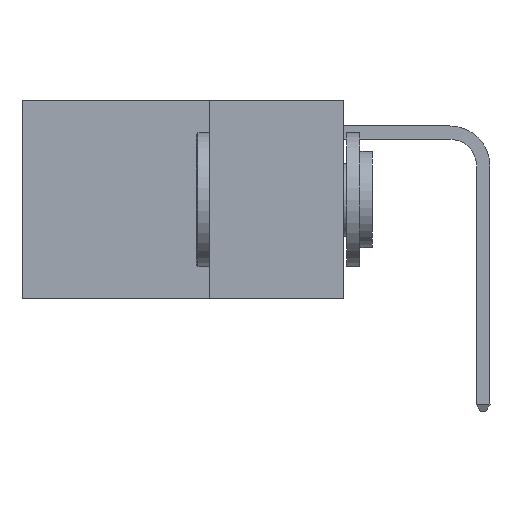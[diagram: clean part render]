
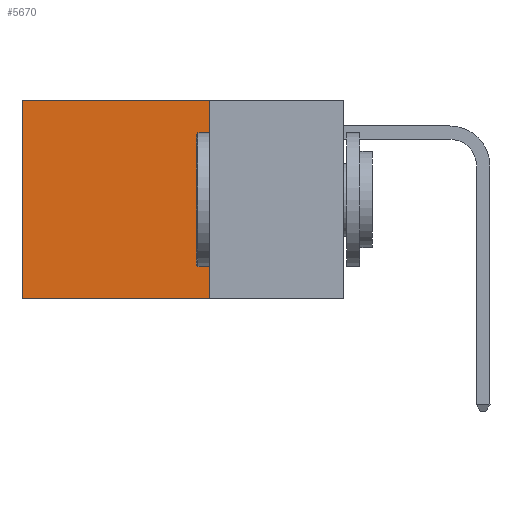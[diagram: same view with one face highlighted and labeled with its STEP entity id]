
A CAD part, left-side view. The second image highlights one B-rep face of the part: STEP entity #5670.
In plain terms, the highlighted planar face has unit normal (-1, 0, 0).
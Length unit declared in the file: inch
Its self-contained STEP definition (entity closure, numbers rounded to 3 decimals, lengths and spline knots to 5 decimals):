
#886 = DIRECTION ( 'NONE',  ( 0., 0., -1. ) ) ;
#1220 = EDGE_CURVE ( 'NONE', #5242, #13661, #16678, .T. ) ;
#1494 = CARTESIAN_POINT ( 'NONE',  ( 0.2625, 0.6, -0.37 ) ) ;
#1855 = FACE_OUTER_BOUND ( 'NONE', #3668, .T. ) ;
#3451 = ORIENTED_EDGE ( 'NONE', *, *, #4221, .T. ) ;
#3668 = EDGE_LOOP ( 'NONE', ( #5160, #16306, #18727, #3451 ) ) ;
#4221 = EDGE_CURVE ( 'NONE', #19881, #21653, #9118, .T. ) ;
#4282 = VECTOR ( 'NONE', #22397, 39.37008 ) ;
#5160 = ORIENTED_EDGE ( 'NONE', *, *, #14125, .T. ) ;
#5242 = VERTEX_POINT ( 'NONE', #20139 ) ;
#5670 = ADVANCED_FACE ( 'NONE', ( #1855 ), #11281, .F. ) ;
#5891 = CARTESIAN_POINT ( 'NONE',  ( 0.2625, 0.25, 0. ) ) ;
#5895 = DIRECTION ( 'NONE',  ( 1., 0., 0. ) ) ;
#7608 = CARTESIAN_POINT ( 'NONE',  ( 0.2625, 0.25, -0.37 ) ) ;
#8099 = LINE ( 'NONE', #20330, #16848 ) ;
#8578 = CARTESIAN_POINT ( 'NONE',  ( 0.2625, 0.25, 0. ) ) ;
#8615 = EDGE_CURVE ( 'NONE', #19881, #5242, #8099, .T. ) ;
#9118 = LINE ( 'NONE', #8578, #4282 ) ;
#10385 = DIRECTION ( 'NONE',  ( 0., 1., 0. ) ) ;
#10437 = LINE ( 'NONE', #22069, #15049 ) ;
#11281 = PLANE ( 'NONE',  #16827 ) ;
#13661 = VERTEX_POINT ( 'NONE', #1494 ) ;
#14125 = EDGE_CURVE ( 'NONE', #21653, #13661, #10437, .T. ) ;
#15049 = VECTOR ( 'NONE', #886, 39.37008 ) ;
#16159 = VECTOR ( 'NONE', #10385, 39.37008 ) ;
#16306 = ORIENTED_EDGE ( 'NONE', *, *, #1220, .F. ) ;
#16457 = CARTESIAN_POINT ( 'NONE',  ( 0.2625, 0.25, 0. ) ) ;
#16563 = CARTESIAN_POINT ( 'NONE',  ( 0.2625, 0.6, 0. ) ) ;
#16678 = LINE ( 'NONE', #7608, #16159 ) ;
#16827 = AXIS2_PLACEMENT_3D ( 'NONE', #16457, #5895, #18172 ) ;
#16848 = VECTOR ( 'NONE', #22030, 39.37008 ) ;
#18172 = DIRECTION ( 'NONE',  ( 0., 0., -1. ) ) ;
#18727 = ORIENTED_EDGE ( 'NONE', *, *, #8615, .F. ) ;
#19881 = VERTEX_POINT ( 'NONE', #5891 ) ;
#20139 = CARTESIAN_POINT ( 'NONE',  ( 0.2625, 0.25, -0.37 ) ) ;
#20330 = CARTESIAN_POINT ( 'NONE',  ( 0.2625, 0.25, 0. ) ) ;
#21653 = VERTEX_POINT ( 'NONE', #16563 ) ;
#22030 = DIRECTION ( 'NONE',  ( 0., 0., -1. ) ) ;
#22069 = CARTESIAN_POINT ( 'NONE',  ( 0.2625, 0.6, 0. ) ) ;
#22397 = DIRECTION ( 'NONE',  ( 0., 1., 0. ) ) ;
